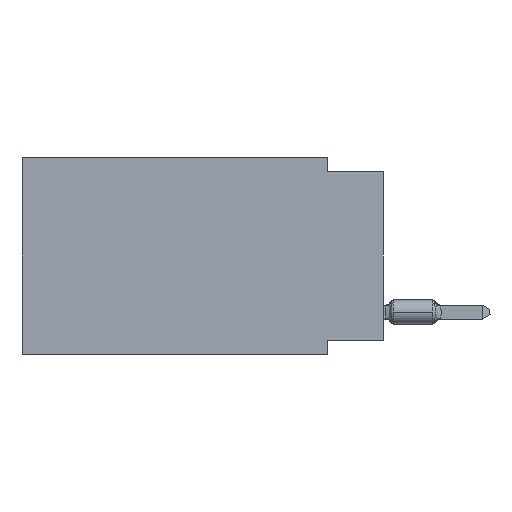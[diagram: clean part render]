
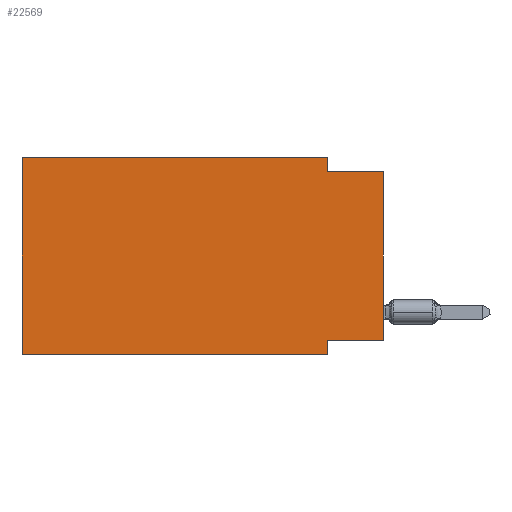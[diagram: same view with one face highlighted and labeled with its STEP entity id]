
A CAD part, left-side view. The second image highlights one B-rep face of the part: STEP entity #22569.
In plain terms, the highlighted planar face has unit normal (-1, 0, 0).
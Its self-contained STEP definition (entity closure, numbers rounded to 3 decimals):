
#13 = VERTEX_POINT ( 'NONE', #46352 ) ;
#238 = ORIENTED_EDGE ( 'NONE', *, *, #23680, .T. ) ;
#1380 = VECTOR ( 'NONE', #2507, 1000. ) ;
#2203 = VERTEX_POINT ( 'NONE', #6638 ) ;
#2377 = ORIENTED_EDGE ( 'NONE', *, *, #13478, .F. ) ;
#2507 = DIRECTION ( 'NONE',  ( 0., 1., 0. ) ) ;
#2683 = ORIENTED_EDGE ( 'NONE', *, *, #40212, .F. ) ;
#3115 = EDGE_CURVE ( 'NONE', #29569, #19876, #38768, .T. ) ;
#5332 = CARTESIAN_POINT ( 'NONE',  ( 0., 2.54, 0. ) ) ;
#5577 = LINE ( 'NONE', #8885, #43761 ) ;
#5969 = VECTOR ( 'NONE', #37680, 1000. ) ;
#6638 = CARTESIAN_POINT ( 'NONE',  ( 0., 0., -0.635 ) ) ;
#7051 = LINE ( 'NONE', #21454, #10613 ) ;
#8885 = CARTESIAN_POINT ( 'NONE',  ( 0., 16.383, 0. ) ) ;
#9469 = ORIENTED_EDGE ( 'NONE', *, *, #43649, .F. ) ;
#10613 = VECTOR ( 'NONE', #35861, 1000. ) ;
#11453 = CARTESIAN_POINT ( 'NONE',  ( 0., 16.383, -8.89 ) ) ;
#11510 = FACE_OUTER_BOUND ( 'NONE', #32581, .T. ) ;
#13478 = EDGE_CURVE ( 'NONE', #13, #29569, #27755, .T. ) ;
#13745 = LINE ( 'NONE', #27916, #37073 ) ;
#13945 = CARTESIAN_POINT ( 'NONE',  ( 0., 2.54, -8.89 ) ) ;
#14566 = VERTEX_POINT ( 'NONE', #43958 ) ;
#14752 = DIRECTION ( 'NONE',  ( 0., -1., 0. ) ) ;
#15809 = LINE ( 'NONE', #37303, #41638 ) ;
#17405 = AXIS2_PLACEMENT_3D ( 'NONE', #40320, #33465, #22371 ) ;
#18653 = EDGE_CURVE ( 'NONE', #34323, #14566, #44291, .T. ) ;
#19757 = VECTOR ( 'NONE', #14752, 1000. ) ;
#19876 = VERTEX_POINT ( 'NONE', #34840 ) ;
#19907 = CARTESIAN_POINT ( 'NONE',  ( 0., 2.54, -8.255 ) ) ;
#20436 = CARTESIAN_POINT ( 'NONE',  ( 0., 0., -8.255 ) ) ;
#21454 = CARTESIAN_POINT ( 'NONE',  ( 0., 0., 0. ) ) ;
#22371 = DIRECTION ( 'NONE',  ( 0., 0., -1. ) ) ;
#22569 = ADVANCED_FACE ( 'NONE', ( #11510 ), #25926, .F. ) ;
#23298 = DIRECTION ( 'NONE',  ( 0., -1., 0. ) ) ;
#23680 = EDGE_CURVE ( 'NONE', #30208, #19876, #32705, .T. ) ;
#24617 = EDGE_CURVE ( 'NONE', #14566, #2203, #13745, .T. ) ;
#24669 = CARTESIAN_POINT ( 'NONE',  ( 0., 2.54, 0. ) ) ;
#25926 = PLANE ( 'NONE',  #17405 ) ;
#27439 = DIRECTION ( 'NONE',  ( 0., -1., 0. ) ) ;
#27755 = LINE ( 'NONE', #20436, #1380 ) ;
#27916 = CARTESIAN_POINT ( 'NONE',  ( 0., 0., -0.635 ) ) ;
#29569 = VERTEX_POINT ( 'NONE', #19907 ) ;
#30208 = VERTEX_POINT ( 'NONE', #32058 ) ;
#30212 = DIRECTION ( 'NONE',  ( 0., 0., 1. ) ) ;
#31681 = VERTEX_POINT ( 'NONE', #35365 ) ;
#32058 = CARTESIAN_POINT ( 'NONE',  ( 0., 16.383, -8.89 ) ) ;
#32581 = EDGE_LOOP ( 'NONE', ( #44661, #41256, #37607, #2683, #9469, #238, #38427, #2377 ) ) ;
#32705 = LINE ( 'NONE', #11453, #19757 ) ;
#33465 = DIRECTION ( 'NONE',  ( 1., 0., 0. ) ) ;
#34063 = EDGE_CURVE ( 'NONE', #13, #2203, #7051, .T. ) ;
#34323 = VERTEX_POINT ( 'NONE', #24669 ) ;
#34840 = CARTESIAN_POINT ( 'NONE',  ( 0., 2.54, -8.89 ) ) ;
#35365 = CARTESIAN_POINT ( 'NONE',  ( 0., 16.383, 0. ) ) ;
#35861 = DIRECTION ( 'NONE',  ( 0., 0., 1. ) ) ;
#36265 = VECTOR ( 'NONE', #39235, 1000. ) ;
#37073 = VECTOR ( 'NONE', #27439, 1000. ) ;
#37303 = CARTESIAN_POINT ( 'NONE',  ( 0., 16.383, 0. ) ) ;
#37607 = ORIENTED_EDGE ( 'NONE', *, *, #18653, .F. ) ;
#37680 = DIRECTION ( 'NONE',  ( 0., 0., -1. ) ) ;
#38427 = ORIENTED_EDGE ( 'NONE', *, *, #3115, .F. ) ;
#38768 = LINE ( 'NONE', #13945, #36265 ) ;
#39235 = DIRECTION ( 'NONE',  ( 0., 0., -1. ) ) ;
#40212 = EDGE_CURVE ( 'NONE', #31681, #34323, #5577, .T. ) ;
#40320 = CARTESIAN_POINT ( 'NONE',  ( 0., 16.383, 0. ) ) ;
#41256 = ORIENTED_EDGE ( 'NONE', *, *, #24617, .F. ) ;
#41638 = VECTOR ( 'NONE', #30212, 1000. ) ;
#43649 = EDGE_CURVE ( 'NONE', #30208, #31681, #15809, .T. ) ;
#43761 = VECTOR ( 'NONE', #23298, 1000. ) ;
#43958 = CARTESIAN_POINT ( 'NONE',  ( 0., 2.54, -0.635 ) ) ;
#44291 = LINE ( 'NONE', #5332, #5969 ) ;
#44661 = ORIENTED_EDGE ( 'NONE', *, *, #34063, .T. ) ;
#46352 = CARTESIAN_POINT ( 'NONE',  ( 0., 0., -8.255 ) ) ;
